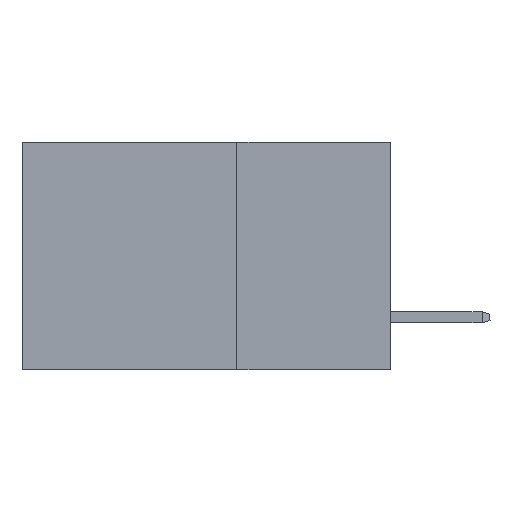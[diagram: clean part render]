
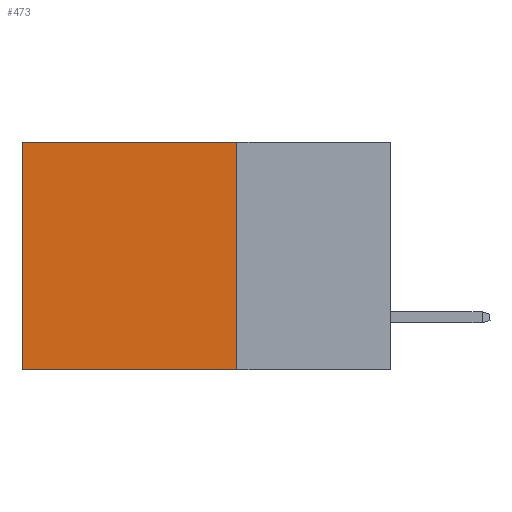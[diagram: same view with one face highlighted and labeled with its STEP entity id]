
A CAD part, left-side view. The second image highlights one B-rep face of the part: STEP entity #473.
In plain terms, the highlighted planar face has unit normal (-1, 0, 0).
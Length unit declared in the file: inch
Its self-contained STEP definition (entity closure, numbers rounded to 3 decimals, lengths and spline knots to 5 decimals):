
#196 = PLANE ( 'NONE',  #9600 ) ;
#368 = CARTESIAN_POINT ( 'NONE',  ( 0.2875, 0.6, 0. ) ) ;
#406 = CARTESIAN_POINT ( 'NONE',  ( 0.2875, 0.25, 0. ) ) ;
#473 = ADVANCED_FACE ( 'NONE', ( #6832 ), #196, .F. ) ;
#1585 = DIRECTION ( 'NONE',  ( 0., 0., -1. ) ) ;
#1626 = EDGE_CURVE ( 'NONE', #6712, #5019, #13838, .T. ) ;
#1676 = EDGE_LOOP ( 'NONE', ( #10318, #1822, #8134, #2571 ) ) ;
#1714 = CARTESIAN_POINT ( 'NONE',  ( 0.2875, 0.25, 0. ) ) ;
#1822 = ORIENTED_EDGE ( 'NONE', *, *, #14402, .F. ) ;
#2111 = CARTESIAN_POINT ( 'NONE',  ( 0.2875, 0.6, -0.37 ) ) ;
#2129 = EDGE_CURVE ( 'NONE', #6712, #7558, #4207, .T. ) ;
#2451 = CARTESIAN_POINT ( 'NONE',  ( 0.2875, 0.25, 0. ) ) ;
#2571 = ORIENTED_EDGE ( 'NONE', *, *, #1626, .T. ) ;
#2824 = LINE ( 'NONE', #368, #13743 ) ;
#3099 = VECTOR ( 'NONE', #10264, 39.37008 ) ;
#4207 = LINE ( 'NONE', #2451, #3099 ) ;
#5019 = VERTEX_POINT ( 'NONE', #13305 ) ;
#5247 = VECTOR ( 'NONE', #11526, 39.37008 ) ;
#6638 = VECTOR ( 'NONE', #8458, 39.37008 ) ;
#6712 = VERTEX_POINT ( 'NONE', #1714 ) ;
#6832 = FACE_OUTER_BOUND ( 'NONE', #1676, .T. ) ;
#7558 = VERTEX_POINT ( 'NONE', #14228 ) ;
#7675 = DIRECTION ( 'NONE',  ( 0., 0., -1. ) ) ;
#8134 = ORIENTED_EDGE ( 'NONE', *, *, #2129, .F. ) ;
#8458 = DIRECTION ( 'NONE',  ( 0., 1., 0. ) ) ;
#8761 = EDGE_CURVE ( 'NONE', #5019, #9103, #2824, .T. ) ;
#9103 = VERTEX_POINT ( 'NONE', #2111 ) ;
#9505 = LINE ( 'NONE', #13821, #6638 ) ;
#9600 = AXIS2_PLACEMENT_3D ( 'NONE', #406, #13344, #7675 ) ;
#10264 = DIRECTION ( 'NONE',  ( 0., 0., -1. ) ) ;
#10318 = ORIENTED_EDGE ( 'NONE', *, *, #8761, .T. ) ;
#10381 = CARTESIAN_POINT ( 'NONE',  ( 0.2875, 0.25, 0. ) ) ;
#11526 = DIRECTION ( 'NONE',  ( 0., 1., 0. ) ) ;
#13305 = CARTESIAN_POINT ( 'NONE',  ( 0.2875, 0.6, 0. ) ) ;
#13344 = DIRECTION ( 'NONE',  ( 1., 0., 0. ) ) ;
#13743 = VECTOR ( 'NONE', #1585, 39.37008 ) ;
#13821 = CARTESIAN_POINT ( 'NONE',  ( 0.2875, 0.25, -0.37 ) ) ;
#13838 = LINE ( 'NONE', #10381, #5247 ) ;
#14228 = CARTESIAN_POINT ( 'NONE',  ( 0.2875, 0.25, -0.37 ) ) ;
#14402 = EDGE_CURVE ( 'NONE', #7558, #9103, #9505, .T. ) ;
